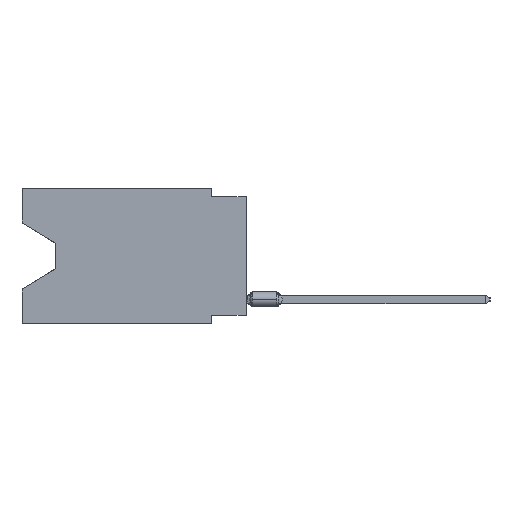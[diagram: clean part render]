
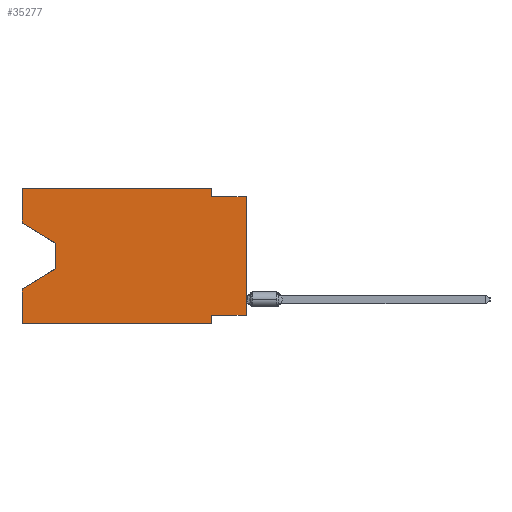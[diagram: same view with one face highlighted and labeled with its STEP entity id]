
A CAD part, left-side view. The second image highlights one B-rep face of the part: STEP entity #35277.
In plain terms, the highlighted planar face has unit normal (-1, 0, 0).
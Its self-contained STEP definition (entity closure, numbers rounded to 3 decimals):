
#562 = ORIENTED_EDGE ( 'NONE', *, *, #31638, .F. ) ;
#989 = ORIENTED_EDGE ( 'NONE', *, *, #1104, .F. ) ;
#1104 = EDGE_CURVE ( 'NONE', #33853, #26682, #6398, .T. ) ;
#1620 = PLANE ( 'NONE',  #17988 ) ;
#2128 = VECTOR ( 'NONE', #25723, 1000. ) ;
#2573 = CARTESIAN_POINT ( 'NONE',  ( 0., 16.383, -2.546 ) ) ;
#3198 = LINE ( 'NONE', #22092, #40280 ) ;
#4097 = VERTEX_POINT ( 'NONE', #14759 ) ;
#4783 = VECTOR ( 'NONE', #30182, 1000. ) ;
#4918 = CARTESIAN_POINT ( 'NONE',  ( 0., 2.54, -9.271 ) ) ;
#5143 = FACE_OUTER_BOUND ( 'NONE', #10316, .T. ) ;
#5191 = VECTOR ( 'NONE', #25217, 1000. ) ;
#5226 = LINE ( 'NONE', #16564, #48709 ) ;
#5248 = CARTESIAN_POINT ( 'NONE',  ( 0., 16.383, 0. ) ) ;
#5553 = LINE ( 'NONE', #17399, #5191 ) ;
#5706 = EDGE_CURVE ( 'NONE', #28606, #7237, #41137, .T. ) ;
#6398 = LINE ( 'NONE', #28574, #6461 ) ;
#6451 = DIRECTION ( 'NONE',  ( 0., 0., 1. ) ) ;
#6461 = VECTOR ( 'NONE', #39920, 1000. ) ;
#6778 = CARTESIAN_POINT ( 'NONE',  ( 0., 2.54, 0. ) ) ;
#6944 = EDGE_CURVE ( 'NONE', #28606, #27172, #35703, .T. ) ;
#7237 = VERTEX_POINT ( 'NONE', #4918 ) ;
#7404 = LINE ( 'NONE', #10416, #22722 ) ;
#9018 = CARTESIAN_POINT ( 'NONE',  ( 0., 2.54, 0. ) ) ;
#9297 = LINE ( 'NONE', #20643, #38757 ) ;
#10091 = ORIENTED_EDGE ( 'NONE', *, *, #5706, .F. ) ;
#10178 = VECTOR ( 'NONE', #6451, 1000. ) ;
#10308 = ORIENTED_EDGE ( 'NONE', *, *, #34290, .T. ) ;
#10316 = EDGE_LOOP ( 'NONE', ( #34885, #35977, #28469, #30988, #10308, #562, #10091, #26935, #47683, #43918, #15670, #989 ) ) ;
#10349 = LINE ( 'NONE', #2573, #2128 ) ;
#10416 = CARTESIAN_POINT ( 'NONE',  ( 0., 13.97, -5.893 ) ) ;
#10574 = EDGE_CURVE ( 'NONE', #12178, #27172, #3198, .T. ) ;
#11688 = VECTOR ( 'NONE', #18224, 1000. ) ;
#12144 = EDGE_CURVE ( 'NONE', #32573, #46979, #7404, .T. ) ;
#12178 = VERTEX_POINT ( 'NONE', #18238 ) ;
#14759 = CARTESIAN_POINT ( 'NONE',  ( 0., 2.54, -9.906 ) ) ;
#15670 = ORIENTED_EDGE ( 'NONE', *, *, #33153, .F. ) ;
#16564 = CARTESIAN_POINT ( 'NONE',  ( 0., 13.97, -4.013 ) ) ;
#17136 = CARTESIAN_POINT ( 'NONE',  ( 0., 16.383, -9.906 ) ) ;
#17399 = CARTESIAN_POINT ( 'NONE',  ( 0., 16.383, 0. ) ) ;
#17559 = CARTESIAN_POINT ( 'NONE',  ( 0., 0., 0. ) ) ;
#17988 = AXIS2_PLACEMENT_3D ( 'NONE', #35853, #24556, #39889 ) ;
#18224 = DIRECTION ( 'NONE',  ( 0., 1., 0. ) ) ;
#18238 = CARTESIAN_POINT ( 'NONE',  ( 0., 2.54, -0.635 ) ) ;
#18389 = LINE ( 'NONE', #29956, #37814 ) ;
#18715 = CARTESIAN_POINT ( 'NONE',  ( 0., 16.383, -7.36 ) ) ;
#19533 = VECTOR ( 'NONE', #34566, 1000. ) ;
#20208 = EDGE_CURVE ( 'NONE', #20508, #12178, #41527, .T. ) ;
#20508 = VERTEX_POINT ( 'NONE', #9018 ) ;
#20643 = CARTESIAN_POINT ( 'NONE',  ( 0., 16.383, 0. ) ) ;
#22092 = CARTESIAN_POINT ( 'NONE',  ( 0., 0., -0.635 ) ) ;
#22722 = VECTOR ( 'NONE', #44684, 1000. ) ;
#23315 = CARTESIAN_POINT ( 'NONE',  ( 0., 0., -0.635 ) ) ;
#24394 = DIRECTION ( 'NONE',  ( 0., 0., -1. ) ) ;
#24556 = DIRECTION ( 'NONE',  ( 1., 0., 0. ) ) ;
#25217 = DIRECTION ( 'NONE',  ( 0., 0., 1. ) ) ;
#25723 = DIRECTION ( 'NONE',  ( 0., -0.855, -0.519 ) ) ;
#26042 = EDGE_CURVE ( 'NONE', #29413, #46979, #5553, .T. ) ;
#26106 = DIRECTION ( 'NONE',  ( 0., -1., 0. ) ) ;
#26682 = VERTEX_POINT ( 'NONE', #5248 ) ;
#26935 = ORIENTED_EDGE ( 'NONE', *, *, #6944, .T. ) ;
#27172 = VERTEX_POINT ( 'NONE', #23315 ) ;
#28469 = ORIENTED_EDGE ( 'NONE', *, *, #12144, .T. ) ;
#28574 = CARTESIAN_POINT ( 'NONE',  ( 0., 16.383, 0. ) ) ;
#28606 = VERTEX_POINT ( 'NONE', #47716 ) ;
#29413 = VERTEX_POINT ( 'NONE', #17136 ) ;
#29956 = CARTESIAN_POINT ( 'NONE',  ( 0., 2.54, -9.906 ) ) ;
#30182 = DIRECTION ( 'NONE',  ( 0., 0., -1. ) ) ;
#30988 = ORIENTED_EDGE ( 'NONE', *, *, #26042, .F. ) ;
#31638 = EDGE_CURVE ( 'NONE', #7237, #4097, #18389, .T. ) ;
#32573 = VERTEX_POINT ( 'NONE', #44222 ) ;
#33153 = EDGE_CURVE ( 'NONE', #26682, #20508, #9297, .T. ) ;
#33853 = VERTEX_POINT ( 'NONE', #41438 ) ;
#34078 = CARTESIAN_POINT ( 'NONE',  ( 0., 16.383, -9.906 ) ) ;
#34290 = EDGE_CURVE ( 'NONE', #29413, #4097, #45399, .T. ) ;
#34566 = DIRECTION ( 'NONE',  ( 0., -1., 0. ) ) ;
#34885 = ORIENTED_EDGE ( 'NONE', *, *, #37000, .T. ) ;
#35277 = ADVANCED_FACE ( 'NONE', ( #5143 ), #1620, .F. ) ;
#35703 = LINE ( 'NONE', #17559, #10178 ) ;
#35853 = CARTESIAN_POINT ( 'NONE',  ( 0., 16.383, 0. ) ) ;
#35977 = ORIENTED_EDGE ( 'NONE', *, *, #37701, .T. ) ;
#37000 = EDGE_CURVE ( 'NONE', #33853, #39445, #10349, .T. ) ;
#37600 = CARTESIAN_POINT ( 'NONE',  ( 0., 0., -9.271 ) ) ;
#37701 = EDGE_CURVE ( 'NONE', #39445, #32573, #5226, .T. ) ;
#37814 = VECTOR ( 'NONE', #40802, 1000. ) ;
#38757 = VECTOR ( 'NONE', #39770, 1000. ) ;
#39445 = VERTEX_POINT ( 'NONE', #48335 ) ;
#39770 = DIRECTION ( 'NONE',  ( 0., -1., 0. ) ) ;
#39889 = DIRECTION ( 'NONE',  ( 0., 0., -1. ) ) ;
#39920 = DIRECTION ( 'NONE',  ( 0., 0., 1. ) ) ;
#40280 = VECTOR ( 'NONE', #26106, 1000. ) ;
#40802 = DIRECTION ( 'NONE',  ( 0., 0., -1. ) ) ;
#41137 = LINE ( 'NONE', #37600, #11688 ) ;
#41438 = CARTESIAN_POINT ( 'NONE',  ( 0., 16.383, -2.546 ) ) ;
#41527 = LINE ( 'NONE', #6778, #4783 ) ;
#43918 = ORIENTED_EDGE ( 'NONE', *, *, #20208, .F. ) ;
#44222 = CARTESIAN_POINT ( 'NONE',  ( 0., 13.97, -5.893 ) ) ;
#44684 = DIRECTION ( 'NONE',  ( 0., 0.855, -0.519 ) ) ;
#45399 = LINE ( 'NONE', #34078, #19533 ) ;
#46979 = VERTEX_POINT ( 'NONE', #18715 ) ;
#47683 = ORIENTED_EDGE ( 'NONE', *, *, #10574, .F. ) ;
#47716 = CARTESIAN_POINT ( 'NONE',  ( 0., 0., -9.271 ) ) ;
#48335 = CARTESIAN_POINT ( 'NONE',  ( 0., 13.97, -4.013 ) ) ;
#48709 = VECTOR ( 'NONE', #24394, 1000. ) ;
